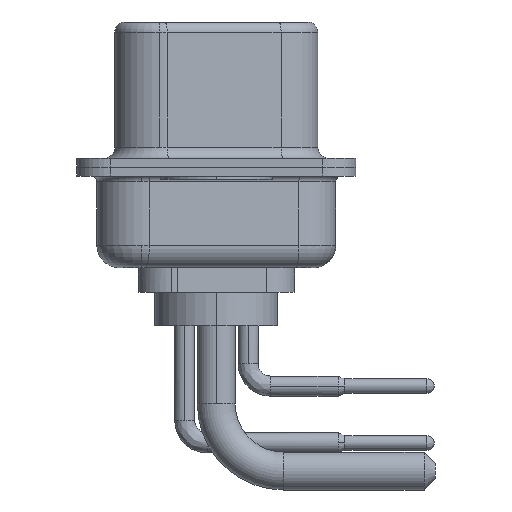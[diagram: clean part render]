
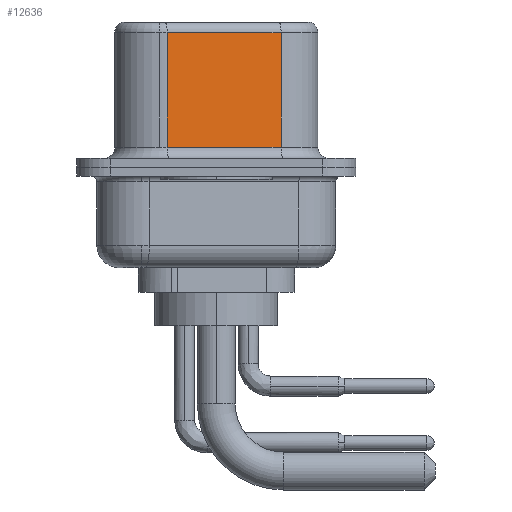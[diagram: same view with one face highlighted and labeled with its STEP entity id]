
A CAD part, left-side view. The second image highlights one B-rep face of the part: STEP entity #12636.
In plain terms, the highlighted planar face has unit normal (-0.985, -0.174, 0).
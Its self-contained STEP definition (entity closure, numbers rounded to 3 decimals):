
#9 = CARTESIAN_POINT ( 'NONE',  ( 4.58, -2.897, 6.02 ) ) ;
#360 = DIRECTION ( 'NONE',  ( -0.174, 0.985, 0. ) ) ;
#644 = EDGE_LOOP ( 'NONE', ( #1267, #6782, #18388, #5836 ) ) ;
#1267 = ORIENTED_EDGE ( 'NONE', *, *, #9091, .F. ) ;
#1436 = LINE ( 'NONE', #4594, #19149 ) ;
#1599 = DIRECTION ( 'NONE',  ( 0., 0., -1. ) ) ;
#1937 = CARTESIAN_POINT ( 'NONE',  ( 4.58, -2.897, 6.52 ) ) ;
#2456 = VECTOR ( 'NONE', #1599, 1000. ) ;
#2613 = CARTESIAN_POINT ( 'NONE',  ( 4.58, -2.897, 0.9 ) ) ;
#2784 = LINE ( 'NONE', #15538, #8790 ) ;
#2957 = LINE ( 'NONE', #17470, #2456 ) ;
#4594 = CARTESIAN_POINT ( 'NONE',  ( 4.58, -2.897, 6.52 ) ) ;
#5076 = FACE_OUTER_BOUND ( 'NONE', #644, .T. ) ;
#5836 = ORIENTED_EDGE ( 'NONE', *, *, #8195, .T. ) ;
#6782 = ORIENTED_EDGE ( 'NONE', *, *, #10288, .T. ) ;
#8195 = EDGE_CURVE ( 'NONE', #12983, #18663, #2784, .T. ) ;
#8326 = DIRECTION ( 'NONE',  ( 0.985, 0.174, 0. ) ) ;
#8790 = VECTOR ( 'NONE', #12200, 1000. ) ;
#8942 = EDGE_CURVE ( 'NONE', #18923, #12983, #2957, .T. ) ;
#9091 = EDGE_CURVE ( 'NONE', #17195, #18663, #1436, .T. ) ;
#10275 = CARTESIAN_POINT ( 'NONE',  ( 4.58, -2.897, 6.02 ) ) ;
#10288 = EDGE_CURVE ( 'NONE', #17195, #18923, #11730, .T. ) ;
#10535 = VECTOR ( 'NONE', #16634, 1000. ) ;
#11433 = CARTESIAN_POINT ( 'NONE',  ( 3.68, 2.203, 0.9 ) ) ;
#11730 = LINE ( 'NONE', #10275, #10535 ) ;
#12200 = DIRECTION ( 'NONE',  ( 0.174, -0.985, 0. ) ) ;
#12636 = ADVANCED_FACE ( 'NONE', ( #5076 ), #14273, .F. ) ;
#12983 = VERTEX_POINT ( 'NONE', #11433 ) ;
#14204 = DIRECTION ( 'NONE',  ( 0., 0., -1. ) ) ;
#14273 = PLANE ( 'NONE',  #15884 ) ;
#14623 = CARTESIAN_POINT ( 'NONE',  ( 3.68, 2.203, 6.02 ) ) ;
#15538 = CARTESIAN_POINT ( 'NONE',  ( 4.58, -2.897, 0.9 ) ) ;
#15884 = AXIS2_PLACEMENT_3D ( 'NONE', #1937, #8326, #360 ) ;
#16634 = DIRECTION ( 'NONE',  ( -0.174, 0.985, 0. ) ) ;
#17195 = VERTEX_POINT ( 'NONE', #9 ) ;
#17470 = CARTESIAN_POINT ( 'NONE',  ( 3.68, 2.203, 6.52 ) ) ;
#18388 = ORIENTED_EDGE ( 'NONE', *, *, #8942, .T. ) ;
#18663 = VERTEX_POINT ( 'NONE', #2613 ) ;
#18923 = VERTEX_POINT ( 'NONE', #14623 ) ;
#19149 = VECTOR ( 'NONE', #14204, 1000. ) ;
